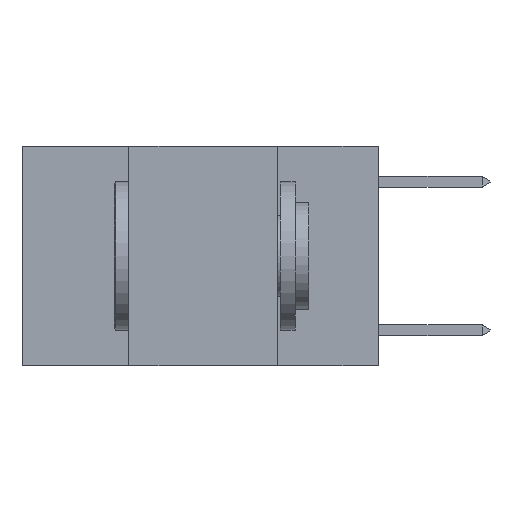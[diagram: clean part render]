
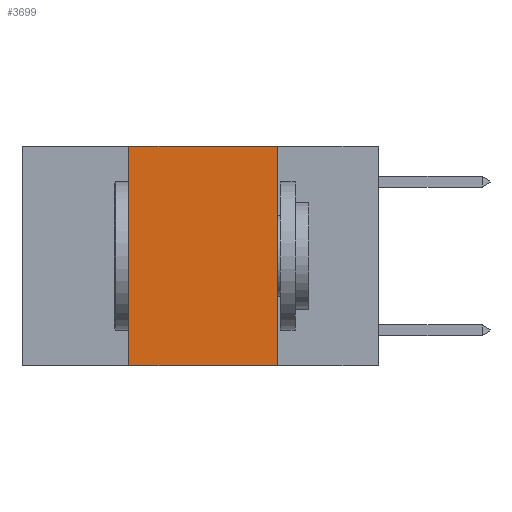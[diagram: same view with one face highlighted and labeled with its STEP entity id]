
A CAD part, left-side view. The second image highlights one B-rep face of the part: STEP entity #3699.
In plain terms, the highlighted planar face has unit normal (-1, 0, 0).
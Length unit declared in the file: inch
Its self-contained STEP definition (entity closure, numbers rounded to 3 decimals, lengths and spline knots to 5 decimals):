
#601 = CARTESIAN_POINT ( 'NONE',  ( 0., 0.17, 0. ) ) ;
#955 = CARTESIAN_POINT ( 'NONE',  ( 0., 0.42, 0. ) ) ;
#1162 = AXIS2_PLACEMENT_3D ( 'NONE', #9418, #13963, #10315 ) ;
#1703 = LINE ( 'NONE', #601, #3768 ) ;
#2328 = DIRECTION ( 'NONE',  ( 0., 0., 1. ) ) ;
#2341 = CARTESIAN_POINT ( 'NONE',  ( 0., 0.6, 0. ) ) ;
#3458 = DIRECTION ( 'NONE',  ( 0., -1., 0. ) ) ;
#3586 = EDGE_CURVE ( 'NONE', #7698, #4396, #11502, .T. ) ;
#3699 = ADVANCED_FACE ( 'NONE', ( #4889 ), #6061, .F. ) ;
#3768 = VECTOR ( 'NONE', #8554, 39.37008 ) ;
#4396 = VERTEX_POINT ( 'NONE', #9057 ) ;
#4736 = VECTOR ( 'NONE', #3458, 39.37008 ) ;
#4889 = FACE_OUTER_BOUND ( 'NONE', #6046, .T. ) ;
#5523 = EDGE_CURVE ( 'NONE', #7426, #4396, #1703, .T. ) ;
#5539 = VERTEX_POINT ( 'NONE', #6125 ) ;
#5579 = DIRECTION ( 'NONE',  ( 0., -1., 0. ) ) ;
#6045 = CARTESIAN_POINT ( 'NONE',  ( 0., 0.42, -0.37 ) ) ;
#6046 = EDGE_LOOP ( 'NONE', ( #10431, #11863, #9993, #13772 ) ) ;
#6061 = PLANE ( 'NONE',  #1162 ) ;
#6125 = CARTESIAN_POINT ( 'NONE',  ( 0., 0.42, 0. ) ) ;
#6607 = LINE ( 'NONE', #955, #14649 ) ;
#7401 = VECTOR ( 'NONE', #5579, 39.37008 ) ;
#7426 = VERTEX_POINT ( 'NONE', #11412 ) ;
#7698 = VERTEX_POINT ( 'NONE', #6045 ) ;
#8554 = DIRECTION ( 'NONE',  ( 0., 0., -1. ) ) ;
#9057 = CARTESIAN_POINT ( 'NONE',  ( 0., 0.17, -0.37 ) ) ;
#9272 = CARTESIAN_POINT ( 'NONE',  ( 0., 0.6, -0.37 ) ) ;
#9418 = CARTESIAN_POINT ( 'NONE',  ( 0., 0.6, 0. ) ) ;
#9993 = ORIENTED_EDGE ( 'NONE', *, *, #12492, .F. ) ;
#10100 = LINE ( 'NONE', #2341, #7401 ) ;
#10271 = EDGE_CURVE ( 'NONE', #5539, #7426, #10100, .T. ) ;
#10315 = DIRECTION ( 'NONE',  ( 0., 0., -1. ) ) ;
#10431 = ORIENTED_EDGE ( 'NONE', *, *, #5523, .F. ) ;
#11412 = CARTESIAN_POINT ( 'NONE',  ( 0., 0.17, 0. ) ) ;
#11502 = LINE ( 'NONE', #9272, #4736 ) ;
#11863 = ORIENTED_EDGE ( 'NONE', *, *, #10271, .F. ) ;
#12492 = EDGE_CURVE ( 'NONE', #7698, #5539, #6607, .T. ) ;
#13772 = ORIENTED_EDGE ( 'NONE', *, *, #3586, .T. ) ;
#13963 = DIRECTION ( 'NONE',  ( 1., 0., 0. ) ) ;
#14649 = VECTOR ( 'NONE', #2328, 39.37008 ) ;
